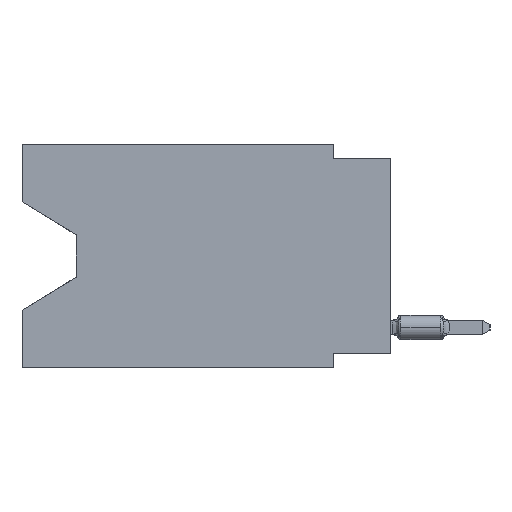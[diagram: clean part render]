
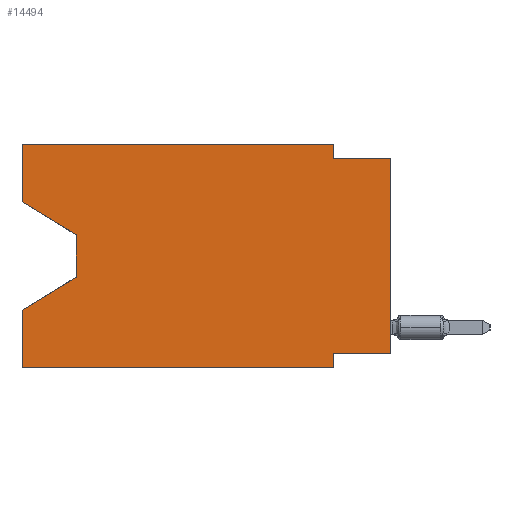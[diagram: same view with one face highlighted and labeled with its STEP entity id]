
A CAD part, left-side view. The second image highlights one B-rep face of the part: STEP entity #14494.
In plain terms, the highlighted planar face has unit normal (-1, 0, 0).
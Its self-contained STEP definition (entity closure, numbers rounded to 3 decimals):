
#300 = AXIS2_PLACEMENT_3D ( 'NONE', #15475, #18733, #460 ) ;
#460 = DIRECTION ( 'NONE',  ( 0., 0., -1. ) ) ;
#631 = ORIENTED_EDGE ( 'NONE', *, *, #16488, .T. ) ;
#1283 = CARTESIAN_POINT ( 'NONE',  ( 0., 13.97, -4.013 ) ) ;
#1521 = DIRECTION ( 'NONE',  ( 0., 1., 0. ) ) ;
#2220 = ORIENTED_EDGE ( 'NONE', *, *, #9189, .F. ) ;
#2526 = CARTESIAN_POINT ( 'NONE',  ( 0., 16.383, -2.546 ) ) ;
#2785 = DIRECTION ( 'NONE',  ( 0., 0., 1. ) ) ;
#2825 = VECTOR ( 'NONE', #1521, 1000. ) ;
#2861 = EDGE_CURVE ( 'NONE', #13045, #8632, #5494, .T. ) ;
#3115 = ORIENTED_EDGE ( 'NONE', *, *, #4439, .T. ) ;
#3355 = DIRECTION ( 'NONE',  ( 0., 0., -1. ) ) ;
#3589 = DIRECTION ( 'NONE',  ( 0., -1., 0. ) ) ;
#3696 = FACE_OUTER_BOUND ( 'NONE', #9673, .T. ) ;
#3785 = CARTESIAN_POINT ( 'NONE',  ( 0., 16.383, -2.546 ) ) ;
#3826 = DIRECTION ( 'NONE',  ( 0., -0.855, -0.519 ) ) ;
#4164 = PLANE ( 'NONE',  #300 ) ;
#4439 = EDGE_CURVE ( 'NONE', #6059, #8632, #13290, .T. ) ;
#4448 = CARTESIAN_POINT ( 'NONE',  ( 0., 0., -0.635 ) ) ;
#4770 = LINE ( 'NONE', #19002, #19784 ) ;
#4992 = EDGE_CURVE ( 'NONE', #15804, #10067, #22533, .T. ) ;
#5116 = VERTEX_POINT ( 'NONE', #9250 ) ;
#5159 = VERTEX_POINT ( 'NONE', #12986 ) ;
#5494 = LINE ( 'NONE', #9118, #23202 ) ;
#6059 = VERTEX_POINT ( 'NONE', #6386 ) ;
#6228 = EDGE_CURVE ( 'NONE', #5159, #13045, #15668, .T. ) ;
#6341 = DIRECTION ( 'NONE',  ( 0., -1., 0. ) ) ;
#6386 = CARTESIAN_POINT ( 'NONE',  ( 0., 0., -9.271 ) ) ;
#6461 = VECTOR ( 'NONE', #6341, 1000. ) ;
#6499 = CARTESIAN_POINT ( 'NONE',  ( 0., 2.54, 0. ) ) ;
#6603 = ORIENTED_EDGE ( 'NONE', *, *, #13120, .F. ) ;
#6659 = LINE ( 'NONE', #1283, #17401 ) ;
#6835 = CARTESIAN_POINT ( 'NONE',  ( 0., 16.383, 0. ) ) ;
#7307 = DIRECTION ( 'NONE',  ( 0., 0., -1. ) ) ;
#7629 = VECTOR ( 'NONE', #3355, 1000. ) ;
#7760 = VERTEX_POINT ( 'NONE', #12366 ) ;
#8259 = ORIENTED_EDGE ( 'NONE', *, *, #2861, .F. ) ;
#8632 = VERTEX_POINT ( 'NONE', #4448 ) ;
#8766 = CARTESIAN_POINT ( 'NONE',  ( 0., 16.383, 0. ) ) ;
#8809 = ORIENTED_EDGE ( 'NONE', *, *, #10209, .T. ) ;
#8878 = DIRECTION ( 'NONE',  ( 0., 0., 1. ) ) ;
#9018 = EDGE_CURVE ( 'NONE', #7760, #10551, #6659, .T. ) ;
#9118 = CARTESIAN_POINT ( 'NONE',  ( 0., 0., -0.635 ) ) ;
#9186 = CARTESIAN_POINT ( 'NONE',  ( 0., 0., -9.271 ) ) ;
#9189 = EDGE_CURVE ( 'NONE', #6059, #16721, #17988, .T. ) ;
#9250 = CARTESIAN_POINT ( 'NONE',  ( 0., 16.383, 0. ) ) ;
#9335 = CARTESIAN_POINT ( 'NONE',  ( 0., 13.97, -5.893 ) ) ;
#9673 = EDGE_LOOP ( 'NONE', ( #631, #16520, #8809, #19957, #20225, #19483, #2220, #3115, #8259, #15809, #6603, #16796 ) ) ;
#9932 = CARTESIAN_POINT ( 'NONE',  ( 0., 0., 0. ) ) ;
#10067 = VERTEX_POINT ( 'NONE', #13447 ) ;
#10209 = EDGE_CURVE ( 'NONE', #10551, #22020, #4770, .T. ) ;
#10551 = VERTEX_POINT ( 'NONE', #9335 ) ;
#10918 = VECTOR ( 'NONE', #3826, 1000. ) ;
#12121 = DIRECTION ( 'NONE',  ( 0., 0.855, -0.519 ) ) ;
#12260 = LINE ( 'NONE', #8766, #13856 ) ;
#12366 = CARTESIAN_POINT ( 'NONE',  ( 0., 13.97, -4.013 ) ) ;
#12678 = EDGE_CURVE ( 'NONE', #14952, #5116, #17579, .T. ) ;
#12986 = CARTESIAN_POINT ( 'NONE',  ( 0., 2.54, 0. ) ) ;
#13045 = VERTEX_POINT ( 'NONE', #17077 ) ;
#13120 = EDGE_CURVE ( 'NONE', #5116, #5159, #16095, .T. ) ;
#13239 = CARTESIAN_POINT ( 'NONE',  ( 0., 16.383, -7.36 ) ) ;
#13290 = LINE ( 'NONE', #9932, #17740 ) ;
#13447 = CARTESIAN_POINT ( 'NONE',  ( 0., 2.54, -9.906 ) ) ;
#13766 = DIRECTION ( 'NONE',  ( 0., 0., 1. ) ) ;
#13778 = DIRECTION ( 'NONE',  ( 0., 0., -1. ) ) ;
#13856 = VECTOR ( 'NONE', #8878, 1000. ) ;
#14052 = CARTESIAN_POINT ( 'NONE',  ( 0., 16.383, 0. ) ) ;
#14494 = ADVANCED_FACE ( 'NONE', ( #3696 ), #4164, .F. ) ;
#14952 = VERTEX_POINT ( 'NONE', #3785 ) ;
#15145 = LINE ( 'NONE', #2526, #10918 ) ;
#15418 = CARTESIAN_POINT ( 'NONE',  ( 0., 16.383, -9.906 ) ) ;
#15475 = CARTESIAN_POINT ( 'NONE',  ( 0., 16.383, 0. ) ) ;
#15668 = LINE ( 'NONE', #6499, #21281 ) ;
#15742 = LINE ( 'NONE', #23434, #7629 ) ;
#15804 = VERTEX_POINT ( 'NONE', #20415 ) ;
#15809 = ORIENTED_EDGE ( 'NONE', *, *, #6228, .F. ) ;
#16093 = CARTESIAN_POINT ( 'NONE',  ( 0., 2.54, -9.271 ) ) ;
#16095 = LINE ( 'NONE', #14052, #6461 ) ;
#16488 = EDGE_CURVE ( 'NONE', #14952, #7760, #15145, .T. ) ;
#16520 = ORIENTED_EDGE ( 'NONE', *, *, #9018, .T. ) ;
#16721 = VERTEX_POINT ( 'NONE', #16093 ) ;
#16796 = ORIENTED_EDGE ( 'NONE', *, *, #12678, .F. ) ;
#17077 = CARTESIAN_POINT ( 'NONE',  ( 0., 2.54, -0.635 ) ) ;
#17401 = VECTOR ( 'NONE', #13778, 1000. ) ;
#17579 = LINE ( 'NONE', #6835, #19169 ) ;
#17740 = VECTOR ( 'NONE', #13766, 1000. ) ;
#17988 = LINE ( 'NONE', #9186, #2825 ) ;
#18733 = DIRECTION ( 'NONE',  ( 1., 0., 0. ) ) ;
#19002 = CARTESIAN_POINT ( 'NONE',  ( 0., 13.97, -5.893 ) ) ;
#19169 = VECTOR ( 'NONE', #2785, 1000. ) ;
#19483 = ORIENTED_EDGE ( 'NONE', *, *, #19509, .F. ) ;
#19509 = EDGE_CURVE ( 'NONE', #16721, #10067, #15742, .T. ) ;
#19784 = VECTOR ( 'NONE', #12121, 1000. ) ;
#19957 = ORIENTED_EDGE ( 'NONE', *, *, #21208, .F. ) ;
#20225 = ORIENTED_EDGE ( 'NONE', *, *, #4992, .T. ) ;
#20415 = CARTESIAN_POINT ( 'NONE',  ( 0., 16.383, -9.906 ) ) ;
#21208 = EDGE_CURVE ( 'NONE', #15804, #22020, #12260, .T. ) ;
#21281 = VECTOR ( 'NONE', #7307, 1000. ) ;
#22020 = VERTEX_POINT ( 'NONE', #13239 ) ;
#22533 = LINE ( 'NONE', #15418, #23339 ) ;
#22755 = DIRECTION ( 'NONE',  ( 0., -1., 0. ) ) ;
#23202 = VECTOR ( 'NONE', #3589, 1000. ) ;
#23339 = VECTOR ( 'NONE', #22755, 1000. ) ;
#23434 = CARTESIAN_POINT ( 'NONE',  ( 0., 2.54, -9.906 ) ) ;
